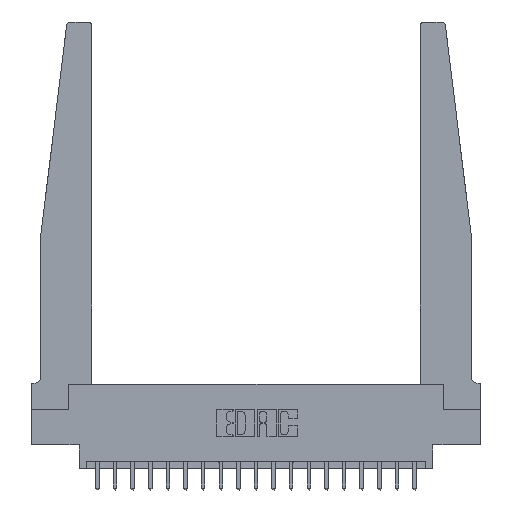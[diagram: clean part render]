
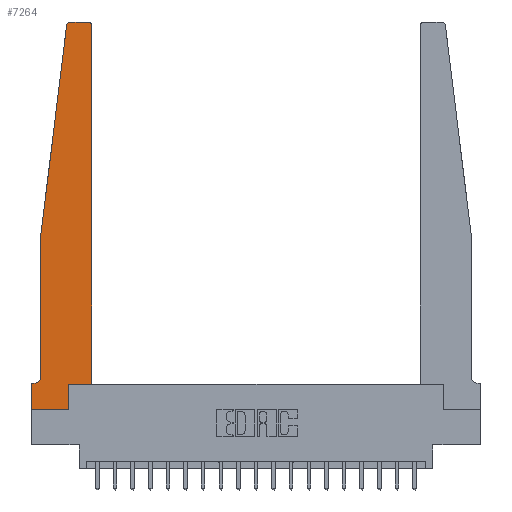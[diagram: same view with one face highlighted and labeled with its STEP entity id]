
A CAD part, top view. The second image highlights one B-rep face of the part: STEP entity #7264.
In plain terms, the highlighted planar face has unit normal (0, 0, 1).
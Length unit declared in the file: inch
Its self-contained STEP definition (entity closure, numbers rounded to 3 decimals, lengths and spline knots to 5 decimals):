
#22 = ORIENTED_EDGE ( 'NONE', *, *, #18348, .T. ) ;
#239 = EDGE_CURVE ( 'NONE', #7594, #13569, #10026, .T. ) ;
#466 = AXIS2_PLACEMENT_3D ( 'NONE', #17451, #2991, #3823 ) ;
#569 = CARTESIAN_POINT ( 'NONE',  ( 0.25, 2.75, 0.37 ) ) ;
#764 = EDGE_CURVE ( 'NONE', #15097, #16999, #5989, .T. ) ;
#1143 = CIRCLE ( 'NONE', #15637, 0.03 ) ;
#2100 = ORIENTED_EDGE ( 'NONE', *, *, #9398, .T. ) ;
#2991 = DIRECTION ( 'NONE',  ( 0., 0., 1. ) ) ;
#3005 = CIRCLE ( 'NONE', #16817, 0.05 ) ;
#3017 = CARTESIAN_POINT ( 'NONE',  ( 0.425, 0.18, 0.37 ) ) ;
#3247 = CARTESIAN_POINT ( 'NONE',  ( 0.27653, 2.72, 0.37 ) ) ;
#3330 = DIRECTION ( 'NONE',  ( -1., 0., 0. ) ) ;
#3397 = EDGE_LOOP ( 'NONE', ( #11530, #2100, #9334, #16213, #5009, #10452, #9861, #13487, #19630, #7979, #22, #17129 ) ) ;
#3453 = DIRECTION ( 'NONE',  ( 1., 0., 0. ) ) ;
#3823 = DIRECTION ( 'NONE',  ( 1., 0., 0. ) ) ;
#3868 = CARTESIAN_POINT ( 'NONE',  ( 0.2605, 0., 0.37 ) ) ;
#3919 = EDGE_CURVE ( 'NONE', #13569, #6197, #17350, .T. ) ;
#4358 = CARTESIAN_POINT ( 'NONE',  ( 0.015, 0.1875, 0.37 ) ) ;
#4398 = AXIS2_PLACEMENT_3D ( 'NONE', #3247, #16023, #3453 ) ;
#4418 = EDGE_CURVE ( 'NONE', #13798, #15097, #6340, .T. ) ;
#4804 = CARTESIAN_POINT ( 'NONE',  ( 0.065, 1.25, 0.37 ) ) ;
#4879 = CARTESIAN_POINT ( 'NONE',  ( 0., 0., 0.37 ) ) ;
#4880 = VECTOR ( 'NONE', #5079, 39.37008 ) ;
#4897 = FACE_OUTER_BOUND ( 'NONE', #3397, .T. ) ;
#5009 = ORIENTED_EDGE ( 'NONE', *, *, #6735, .T. ) ;
#5079 = DIRECTION ( 'NONE',  ( 0., 1., 0. ) ) ;
#5225 = LINE ( 'NONE', #569, #17824 ) ;
#5270 = EDGE_CURVE ( 'NONE', #11001, #11140, #5225, .T. ) ;
#5388 = DIRECTION ( 'NONE',  ( 0., 1., 0. ) ) ;
#5435 = CARTESIAN_POINT ( 'NONE',  ( 0.425, 2.72, 0.37 ) ) ;
#5438 = DIRECTION ( 'NONE',  ( -1., 0., 0. ) ) ;
#5989 = LINE ( 'NONE', #13885, #20759 ) ;
#6197 = VERTEX_POINT ( 'NONE', #13937 ) ;
#6213 = CARTESIAN_POINT ( 'NONE',  ( 0.065, 0.2375, 0.37 ) ) ;
#6309 = VECTOR ( 'NONE', #11404, 39.37008 ) ;
#6340 = LINE ( 'NONE', #19524, #4880 ) ;
#6735 = EDGE_CURVE ( 'NONE', #9534, #7594, #3005, .T. ) ;
#7264 = ADVANCED_FACE ( 'NONE', ( #4897 ), #11007, .T. ) ;
#7582 = EDGE_CURVE ( 'NONE', #13483, #9131, #18498, .T. ) ;
#7594 = VERTEX_POINT ( 'NONE', #4358 ) ;
#7829 = CARTESIAN_POINT ( 'NONE',  ( 0., 0., 0.37 ) ) ;
#7979 = ORIENTED_EDGE ( 'NONE', *, *, #764, .T. ) ;
#8024 = CARTESIAN_POINT ( 'NONE',  ( 0.24675, 2.72367, 0.37 ) ) ;
#8046 = DIRECTION ( 'NONE',  ( 0., -1., 0. ) ) ;
#8068 = CARTESIAN_POINT ( 'NONE',  ( 0.27653, 2.75, 0.37 ) ) ;
#8857 = DIRECTION ( 'NONE',  ( -0.122, -0.992, 0. ) ) ;
#9085 = EDGE_CURVE ( 'NONE', #6197, #13798, #10991, .T. ) ;
#9131 = VERTEX_POINT ( 'NONE', #14467 ) ;
#9139 = DIRECTION ( 'NONE',  ( 0., 0., 1. ) ) ;
#9334 = ORIENTED_EDGE ( 'NONE', *, *, #7582, .T. ) ;
#9398 = EDGE_CURVE ( 'NONE', #11140, #13483, #14833, .T. ) ;
#9534 = VERTEX_POINT ( 'NONE', #6213 ) ;
#9861 = ORIENTED_EDGE ( 'NONE', *, *, #3919, .T. ) ;
#10026 = LINE ( 'NONE', #16176, #13315 ) ;
#10452 = ORIENTED_EDGE ( 'NONE', *, *, #239, .T. ) ;
#10915 = LINE ( 'NONE', #4804, #19574 ) ;
#10991 = LINE ( 'NONE', #4879, #6309 ) ;
#11001 = VERTEX_POINT ( 'NONE', #15391 ) ;
#11007 = PLANE ( 'NONE',  #466 ) ;
#11140 = VERTEX_POINT ( 'NONE', #8068 ) ;
#11404 = DIRECTION ( 'NONE',  ( 1., 0., 0. ) ) ;
#11446 = CARTESIAN_POINT ( 'NONE',  ( 0.015, 0.2375, 0.37 ) ) ;
#11530 = ORIENTED_EDGE ( 'NONE', *, *, #5270, .T. ) ;
#12616 = VECTOR ( 'NONE', #15566, 39.37008 ) ;
#12744 = DIRECTION ( 'NONE',  ( 1., 0., 0. ) ) ;
#12981 = EDGE_CURVE ( 'NONE', #9131, #9534, #10915, .T. ) ;
#13315 = VECTOR ( 'NONE', #16498, 39.37008 ) ;
#13483 = VERTEX_POINT ( 'NONE', #8024 ) ;
#13487 = ORIENTED_EDGE ( 'NONE', *, *, #9085, .T. ) ;
#13569 = VERTEX_POINT ( 'NONE', #20059 ) ;
#13708 = CARTESIAN_POINT ( 'NONE',  ( 0.425, 0.18, 0.37 ) ) ;
#13798 = VERTEX_POINT ( 'NONE', #3868 ) ;
#13885 = CARTESIAN_POINT ( 'NONE',  ( 0.425, 0.18, 0.37 ) ) ;
#13937 = CARTESIAN_POINT ( 'NONE',  ( 0., 0., 0.37 ) ) ;
#14020 = CARTESIAN_POINT ( 'NONE',  ( 0.395, 2.72, 0.37 ) ) ;
#14182 = VERTEX_POINT ( 'NONE', #5435 ) ;
#14467 = CARTESIAN_POINT ( 'NONE',  ( 0.065, 1.25, 0.37 ) ) ;
#14833 = CIRCLE ( 'NONE', #4398, 0.03 ) ;
#15097 = VERTEX_POINT ( 'NONE', #17945 ) ;
#15391 = CARTESIAN_POINT ( 'NONE',  ( 0.395, 2.75, 0.37 ) ) ;
#15434 = CARTESIAN_POINT ( 'NONE',  ( 0.065, 1.25, 0.37 ) ) ;
#15566 = DIRECTION ( 'NONE',  ( 0., -1., 0. ) ) ;
#15637 = AXIS2_PLACEMENT_3D ( 'NONE', #14020, #9139, #12744 ) ;
#15701 = VECTOR ( 'NONE', #5388, 39.37008 ) ;
#16023 = DIRECTION ( 'NONE',  ( 0., 0., 1. ) ) ;
#16176 = CARTESIAN_POINT ( 'NONE',  ( 0.065, 0.1875, 0.37 ) ) ;
#16213 = ORIENTED_EDGE ( 'NONE', *, *, #12981, .T. ) ;
#16498 = DIRECTION ( 'NONE',  ( -1., 0., 0. ) ) ;
#16670 = LINE ( 'NONE', #13708, #15701 ) ;
#16731 = EDGE_CURVE ( 'NONE', #14182, #11001, #1143, .T. ) ;
#16817 = AXIS2_PLACEMENT_3D ( 'NONE', #11446, #17795, #3330 ) ;
#16999 = VERTEX_POINT ( 'NONE', #3017 ) ;
#17129 = ORIENTED_EDGE ( 'NONE', *, *, #16731, .T. ) ;
#17350 = LINE ( 'NONE', #7829, #12616 ) ;
#17451 = CARTESIAN_POINT ( 'NONE',  ( 0., 0.1875, 0.37 ) ) ;
#17795 = DIRECTION ( 'NONE',  ( 0., 0., -1. ) ) ;
#17824 = VECTOR ( 'NONE', #5438, 39.37008 ) ;
#17945 = CARTESIAN_POINT ( 'NONE',  ( 0.2605, 0.18, 0.37 ) ) ;
#18348 = EDGE_CURVE ( 'NONE', #16999, #14182, #16670, .T. ) ;
#18498 = LINE ( 'NONE', #15434, #20034 ) ;
#19524 = CARTESIAN_POINT ( 'NONE',  ( 0.2605, 0.18, 0.37 ) ) ;
#19574 = VECTOR ( 'NONE', #8046, 39.37008 ) ;
#19630 = ORIENTED_EDGE ( 'NONE', *, *, #4418, .T. ) ;
#20034 = VECTOR ( 'NONE', #8857, 39.37008 ) ;
#20059 = CARTESIAN_POINT ( 'NONE',  ( 0., 0.1875, 0.37 ) ) ;
#20437 = DIRECTION ( 'NONE',  ( 1., 0., 0. ) ) ;
#20759 = VECTOR ( 'NONE', #20437, 39.37008 ) ;
